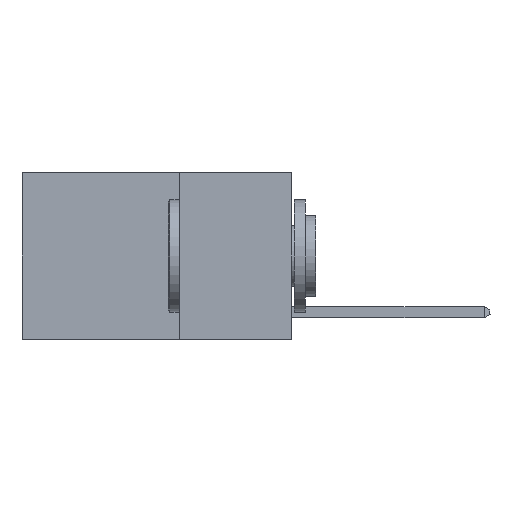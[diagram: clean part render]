
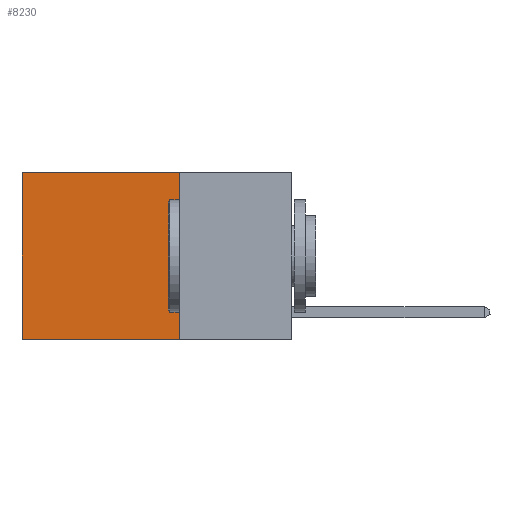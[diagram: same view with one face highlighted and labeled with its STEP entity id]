
A CAD part, left-side view. The second image highlights one B-rep face of the part: STEP entity #8230.
In plain terms, the highlighted planar face has unit normal (-1, 0, 0).
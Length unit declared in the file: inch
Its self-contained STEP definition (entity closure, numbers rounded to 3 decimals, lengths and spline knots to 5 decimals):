
#380 = ORIENTED_EDGE ( 'NONE', *, *, #3180, .F. ) ;
#804 = VECTOR ( 'NONE', #12348, 39.37008 ) ;
#1947 = DIRECTION ( 'NONE',  ( 0., 0., -1. ) ) ;
#2918 = ORIENTED_EDGE ( 'NONE', *, *, #4059, .F. ) ;
#3180 = EDGE_CURVE ( 'NONE', #21239, #7402, #19801, .T. ) ;
#3309 = VECTOR ( 'NONE', #18637, 39.37008 ) ;
#3749 = CARTESIAN_POINT ( 'NONE',  ( 0.2625, 0.25, 0. ) ) ;
#3761 = AXIS2_PLACEMENT_3D ( 'NONE', #3749, #10624, #1947 ) ;
#3863 = PLANE ( 'NONE',  #3761 ) ;
#4014 = VECTOR ( 'NONE', #12264, 39.37008 ) ;
#4059 = EDGE_CURVE ( 'NONE', #7402, #18153, #13534, .T. ) ;
#4194 = CARTESIAN_POINT ( 'NONE',  ( 0.2625, 0.25, 0. ) ) ;
#4824 = CARTESIAN_POINT ( 'NONE',  ( 0.2625, 0.25, -0.37 ) ) ;
#5714 = LINE ( 'NONE', #19520, #4014 ) ;
#5973 = EDGE_LOOP ( 'NONE', ( #18267, #2918, #380, #21164 ) ) ;
#7062 = LINE ( 'NONE', #20842, #804 ) ;
#7402 = VERTEX_POINT ( 'NONE', #20265 ) ;
#8230 = ADVANCED_FACE ( 'NONE', ( #14123 ), #3863, .F. ) ;
#9616 = DIRECTION ( 'NONE',  ( 0., 0., -1. ) ) ;
#10624 = DIRECTION ( 'NONE',  ( 1., 0., 0. ) ) ;
#11282 = VERTEX_POINT ( 'NONE', #21814 ) ;
#12264 = DIRECTION ( 'NONE',  ( 0., 0., -1. ) ) ;
#12309 = VECTOR ( 'NONE', #9616, 39.37008 ) ;
#12348 = DIRECTION ( 'NONE',  ( 0., 1., 0. ) ) ;
#13534 = LINE ( 'NONE', #4824, #3309 ) ;
#13942 = CARTESIAN_POINT ( 'NONE',  ( 0.2625, 0.25, 0. ) ) ;
#14123 = FACE_OUTER_BOUND ( 'NONE', #5973, .T. ) ;
#17767 = EDGE_CURVE ( 'NONE', #11282, #18153, #5714, .T. ) ;
#18153 = VERTEX_POINT ( 'NONE', #19273 ) ;
#18197 = EDGE_CURVE ( 'NONE', #21239, #11282, #7062, .T. ) ;
#18267 = ORIENTED_EDGE ( 'NONE', *, *, #17767, .T. ) ;
#18637 = DIRECTION ( 'NONE',  ( 0., 1., 0. ) ) ;
#19273 = CARTESIAN_POINT ( 'NONE',  ( 0.2625, 0.6, -0.37 ) ) ;
#19520 = CARTESIAN_POINT ( 'NONE',  ( 0.2625, 0.6, 0. ) ) ;
#19801 = LINE ( 'NONE', #4194, #12309 ) ;
#20265 = CARTESIAN_POINT ( 'NONE',  ( 0.2625, 0.25, -0.37 ) ) ;
#20842 = CARTESIAN_POINT ( 'NONE',  ( 0.2625, 0.25, 0. ) ) ;
#21164 = ORIENTED_EDGE ( 'NONE', *, *, #18197, .T. ) ;
#21239 = VERTEX_POINT ( 'NONE', #13942 ) ;
#21814 = CARTESIAN_POINT ( 'NONE',  ( 0.2625, 0.6, 0. ) ) ;
